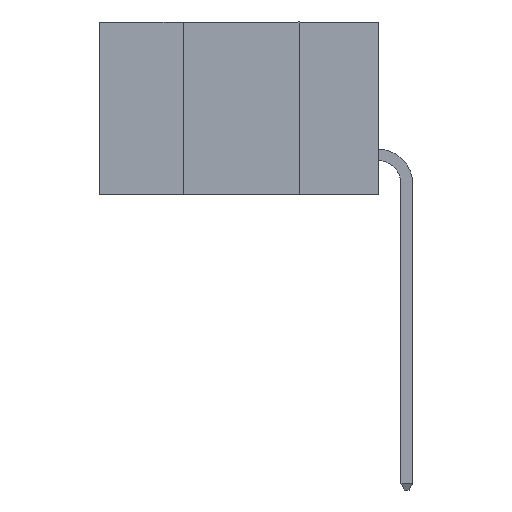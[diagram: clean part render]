
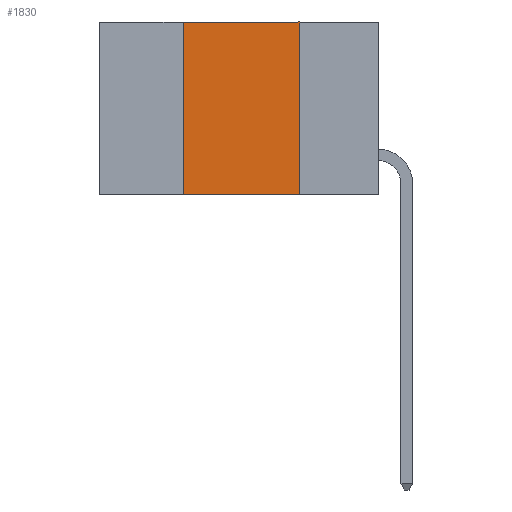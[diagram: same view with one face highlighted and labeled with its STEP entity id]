
A CAD part, left-side view. The second image highlights one B-rep face of the part: STEP entity #1830.
In plain terms, the highlighted planar face has unit normal (-1, 0, 0).
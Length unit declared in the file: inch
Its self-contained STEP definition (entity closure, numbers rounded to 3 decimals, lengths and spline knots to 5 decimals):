
#639 = DIRECTION ( 'NONE',  ( 0., -1., 0. ) ) ;
#1445 = FACE_OUTER_BOUND ( 'NONE', #7189, .T. ) ;
#1481 = CARTESIAN_POINT ( 'NONE',  ( 0., 0.42, 0. ) ) ;
#1830 = ADVANCED_FACE ( 'NONE', ( #1445 ), #15783, .F. ) ;
#1952 = CARTESIAN_POINT ( 'NONE',  ( 0., 0.17, 0. ) ) ;
#2914 = VECTOR ( 'NONE', #6043, 39.37008 ) ;
#2978 = VERTEX_POINT ( 'NONE', #3892 ) ;
#2988 = ORIENTED_EDGE ( 'NONE', *, *, #16905, .F. ) ;
#3882 = CARTESIAN_POINT ( 'NONE',  ( 0., 0.42, -0.37 ) ) ;
#3892 = CARTESIAN_POINT ( 'NONE',  ( 0., 0.17, -0.37 ) ) ;
#3939 = VECTOR ( 'NONE', #5264, 39.37008 ) ;
#4636 = CARTESIAN_POINT ( 'NONE',  ( 0., 0.17, -0.37 ) ) ;
#4711 = VERTEX_POINT ( 'NONE', #14212 ) ;
#5251 = AXIS2_PLACEMENT_3D ( 'NONE', #16306, #15613, #14367 ) ;
#5264 = DIRECTION ( 'NONE',  ( 0., 0., 1. ) ) ;
#6043 = DIRECTION ( 'NONE',  ( 0., 0., -1. ) ) ;
#6308 = VECTOR ( 'NONE', #6952, 39.37008 ) ;
#6339 = EDGE_CURVE ( 'NONE', #14716, #2978, #13910, .T. ) ;
#6890 = CARTESIAN_POINT ( 'NONE',  ( 0., 0.6, 0. ) ) ;
#6952 = DIRECTION ( 'NONE',  ( 0., -1., 0. ) ) ;
#7189 = EDGE_LOOP ( 'NONE', ( #16210, #2988, #9340, #9132 ) ) ;
#7365 = VECTOR ( 'NONE', #639, 39.37008 ) ;
#7794 = LINE ( 'NONE', #17051, #7365 ) ;
#9132 = ORIENTED_EDGE ( 'NONE', *, *, #12503, .T. ) ;
#9340 = ORIENTED_EDGE ( 'NONE', *, *, #16048, .F. ) ;
#10443 = LINE ( 'NONE', #6890, #6308 ) ;
#11596 = VERTEX_POINT ( 'NONE', #1481 ) ;
#11720 = LINE ( 'NONE', #3882, #3939 ) ;
#12503 = EDGE_CURVE ( 'NONE', #4711, #2978, #7794, .T. ) ;
#13910 = LINE ( 'NONE', #4636, #2914 ) ;
#14212 = CARTESIAN_POINT ( 'NONE',  ( 0., 0.42, -0.37 ) ) ;
#14367 = DIRECTION ( 'NONE',  ( 0., 0., -1. ) ) ;
#14716 = VERTEX_POINT ( 'NONE', #1952 ) ;
#15613 = DIRECTION ( 'NONE',  ( 1., 0., 0. ) ) ;
#15783 = PLANE ( 'NONE',  #5251 ) ;
#16048 = EDGE_CURVE ( 'NONE', #4711, #11596, #11720, .T. ) ;
#16210 = ORIENTED_EDGE ( 'NONE', *, *, #6339, .F. ) ;
#16306 = CARTESIAN_POINT ( 'NONE',  ( 0., 0.6, 0. ) ) ;
#16905 = EDGE_CURVE ( 'NONE', #11596, #14716, #10443, .T. ) ;
#17051 = CARTESIAN_POINT ( 'NONE',  ( 0., 0.6, -0.37 ) ) ;
